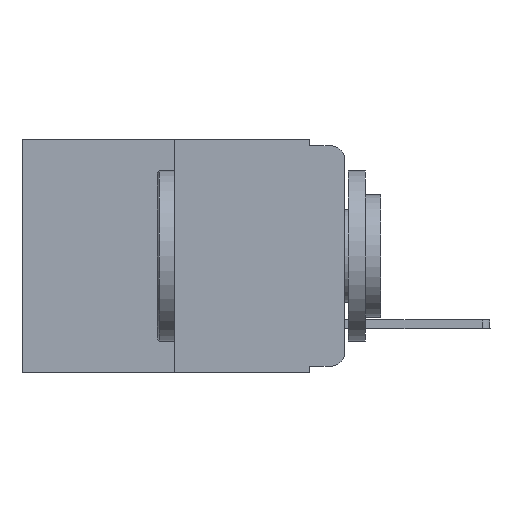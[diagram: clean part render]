
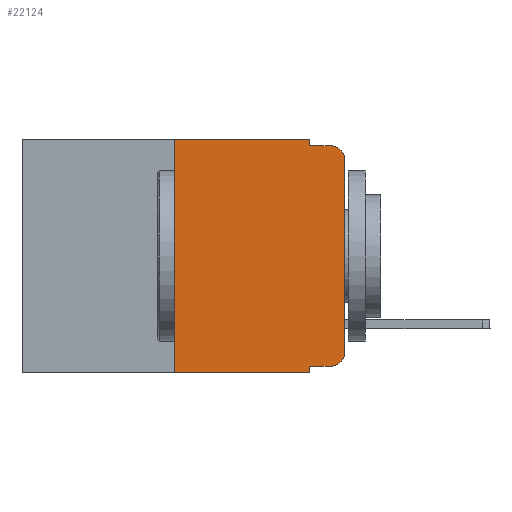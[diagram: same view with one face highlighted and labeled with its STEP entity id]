
A CAD part, left-side view. The second image highlights one B-rep face of the part: STEP entity #22124.
In plain terms, the highlighted planar face has unit normal (-1, 0, 0).
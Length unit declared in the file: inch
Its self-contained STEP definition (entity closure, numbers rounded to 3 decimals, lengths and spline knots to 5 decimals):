
#233 = LINE ( 'NONE', #1304, #16641 ) ;
#449 = CIRCLE ( 'NONE', #2284, 0.02 ) ;
#474 = VERTEX_POINT ( 'NONE', #22057 ) ;
#718 = ORIENTED_EDGE ( 'NONE', *, *, #19551, .F. ) ;
#771 = CARTESIAN_POINT ( 'NONE',  ( 0., 0.051, 0. ) ) ;
#820 = ORIENTED_EDGE ( 'NONE', *, *, #11929, .T. ) ;
#848 = CARTESIAN_POINT ( 'NONE',  ( 0., 0.051, 0. ) ) ;
#858 = CARTESIAN_POINT ( 'NONE',  ( 0., 0.051, -0.01 ) ) ;
#1251 = VERTEX_POINT ( 'NONE', #17158 ) ;
#1304 = CARTESIAN_POINT ( 'NONE',  ( 0., 0.051, -0.333 ) ) ;
#1916 = EDGE_CURVE ( 'NONE', #1251, #18684, #23130, .T. ) ;
#2217 = CARTESIAN_POINT ( 'NONE',  ( 0., 0.25, -0.343 ) ) ;
#2268 = CARTESIAN_POINT ( 'NONE',  ( 0., 0.473, -0.343 ) ) ;
#2284 = AXIS2_PLACEMENT_3D ( 'NONE', #17686, #22998, #9937 ) ;
#3034 = VERTEX_POINT ( 'NONE', #2217 ) ;
#3412 = LINE ( 'NONE', #2268, #17535 ) ;
#3531 = ORIENTED_EDGE ( 'NONE', *, *, #14633, .T. ) ;
#3985 = CARTESIAN_POINT ( 'NONE',  ( 0., 0.02, -0.01 ) ) ;
#4233 = CIRCLE ( 'NONE', #8133, 0.02 ) ;
#4594 = VERTEX_POINT ( 'NONE', #23508 ) ;
#5028 = VERTEX_POINT ( 'NONE', #7505 ) ;
#5081 = PLANE ( 'NONE',  #6099 ) ;
#5226 = DIRECTION ( 'NONE',  ( 1., 0., 0. ) ) ;
#5982 = CARTESIAN_POINT ( 'NONE',  ( 0., 0.473, 0. ) ) ;
#6099 = AXIS2_PLACEMENT_3D ( 'NONE', #13432, #5226, #8770 ) ;
#6100 = DIRECTION ( 'NONE',  ( -1., 0., 0. ) ) ;
#6315 = ORIENTED_EDGE ( 'NONE', *, *, #8791, .F. ) ;
#6848 = VERTEX_POINT ( 'NONE', #3985 ) ;
#6856 = CARTESIAN_POINT ( 'NONE',  ( 0., 0., -0.03 ) ) ;
#6919 = EDGE_CURVE ( 'NONE', #474, #1251, #12435, .T. ) ;
#7505 = CARTESIAN_POINT ( 'NONE',  ( 0., 0., -0.313 ) ) ;
#7773 = DIRECTION ( 'NONE',  ( 0., -1., 0. ) ) ;
#7808 = VERTEX_POINT ( 'NONE', #14983 ) ;
#8133 = AXIS2_PLACEMENT_3D ( 'NONE', #17137, #6100, #9895 ) ;
#8562 = ORIENTED_EDGE ( 'NONE', *, *, #12591, .T. ) ;
#8770 = DIRECTION ( 'NONE',  ( 0., 0., -1. ) ) ;
#8789 = ORIENTED_EDGE ( 'NONE', *, *, #22427, .T. ) ;
#8791 = EDGE_CURVE ( 'NONE', #3034, #474, #13846, .T. ) ;
#8954 = VECTOR ( 'NONE', #19893, 39.37008 ) ;
#9895 = DIRECTION ( 'NONE',  ( 0., 0., -1. ) ) ;
#9937 = DIRECTION ( 'NONE',  ( 0., 0., -1. ) ) ;
#10815 = CARTESIAN_POINT ( 'NONE',  ( 0., 0., 0. ) ) ;
#11022 = EDGE_LOOP ( 'NONE', ( #820, #8562, #18876, #11341, #19457, #6315, #15344, #718, #3531, #8789 ) ) ;
#11085 = VERTEX_POINT ( 'NONE', #12079 ) ;
#11341 = ORIENTED_EDGE ( 'NONE', *, *, #1916, .F. ) ;
#11691 = DIRECTION ( 'NONE',  ( 0., 0., -1. ) ) ;
#11929 = EDGE_CURVE ( 'NONE', #5028, #19697, #21535, .T. ) ;
#12079 = CARTESIAN_POINT ( 'NONE',  ( 0., 0.051, -0.343 ) ) ;
#12435 = LINE ( 'NONE', #5982, #16759 ) ;
#12591 = EDGE_CURVE ( 'NONE', #19697, #6848, #449, .T. ) ;
#12650 = DIRECTION ( 'NONE',  ( 0., 0., 1. ) ) ;
#13432 = CARTESIAN_POINT ( 'NONE',  ( 0., 0.473, 0. ) ) ;
#13846 = LINE ( 'NONE', #14531, #8954 ) ;
#13938 = DIRECTION ( 'NONE',  ( 0., 0., -1. ) ) ;
#14087 = LINE ( 'NONE', #848, #14650 ) ;
#14531 = CARTESIAN_POINT ( 'NONE',  ( 0., 0.25, 0. ) ) ;
#14633 = EDGE_CURVE ( 'NONE', #4594, #7808, #233, .T. ) ;
#14650 = VECTOR ( 'NONE', #13938, 39.37008 ) ;
#14983 = CARTESIAN_POINT ( 'NONE',  ( 0., 0.02, -0.333 ) ) ;
#15344 = ORIENTED_EDGE ( 'NONE', *, *, #21805, .T. ) ;
#15368 = DIRECTION ( 'NONE',  ( 0., -1., 0. ) ) ;
#15933 = DIRECTION ( 'NONE',  ( 0., -1., 0. ) ) ;
#16475 = VECTOR ( 'NONE', #11691, 39.37008 ) ;
#16641 = VECTOR ( 'NONE', #23453, 39.37008 ) ;
#16759 = VECTOR ( 'NONE', #7773, 39.37008 ) ;
#17137 = CARTESIAN_POINT ( 'NONE',  ( 0., 0.02, -0.313 ) ) ;
#17158 = CARTESIAN_POINT ( 'NONE',  ( 0., 0.051, 0. ) ) ;
#17209 = FACE_OUTER_BOUND ( 'NONE', #11022, .T. ) ;
#17507 = VECTOR ( 'NONE', #15933, 39.37008 ) ;
#17535 = VECTOR ( 'NONE', #15368, 39.37008 ) ;
#17686 = CARTESIAN_POINT ( 'NONE',  ( 0., 0.02, -0.03 ) ) ;
#18684 = VERTEX_POINT ( 'NONE', #858 ) ;
#18876 = ORIENTED_EDGE ( 'NONE', *, *, #22113, .F. ) ;
#19457 = ORIENTED_EDGE ( 'NONE', *, *, #6919, .F. ) ;
#19551 = EDGE_CURVE ( 'NONE', #4594, #11085, #14087, .T. ) ;
#19594 = CARTESIAN_POINT ( 'NONE',  ( 0., 0.051, -0.01 ) ) ;
#19697 = VERTEX_POINT ( 'NONE', #6856 ) ;
#19836 = LINE ( 'NONE', #19594, #17507 ) ;
#19893 = DIRECTION ( 'NONE',  ( 0., 0., 1. ) ) ;
#21244 = VECTOR ( 'NONE', #12650, 39.37008 ) ;
#21535 = LINE ( 'NONE', #10815, #21244 ) ;
#21805 = EDGE_CURVE ( 'NONE', #3034, #11085, #3412, .T. ) ;
#22057 = CARTESIAN_POINT ( 'NONE',  ( 0., 0.25, 0. ) ) ;
#22113 = EDGE_CURVE ( 'NONE', #18684, #6848, #19836, .T. ) ;
#22124 = ADVANCED_FACE ( 'NONE', ( #17209 ), #5081, .F. ) ;
#22427 = EDGE_CURVE ( 'NONE', #7808, #5028, #4233, .T. ) ;
#22998 = DIRECTION ( 'NONE',  ( -1., 0., 0. ) ) ;
#23130 = LINE ( 'NONE', #771, #16475 ) ;
#23453 = DIRECTION ( 'NONE',  ( 0., -1., 0. ) ) ;
#23508 = CARTESIAN_POINT ( 'NONE',  ( 0., 0.051, -0.333 ) ) ;
